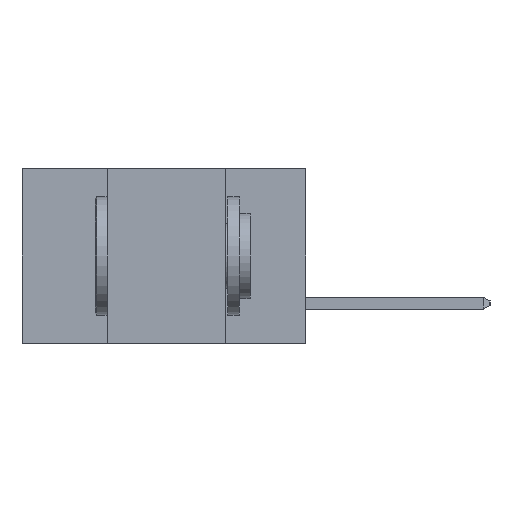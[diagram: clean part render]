
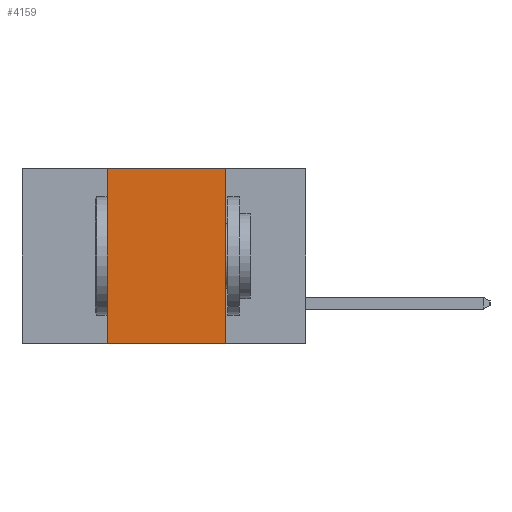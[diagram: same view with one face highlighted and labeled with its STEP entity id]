
A CAD part, left-side view. The second image highlights one B-rep face of the part: STEP entity #4159.
In plain terms, the highlighted planar face has unit normal (-1, 0, 0).
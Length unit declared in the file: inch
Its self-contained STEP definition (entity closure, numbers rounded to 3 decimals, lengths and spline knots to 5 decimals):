
#838 = LINE ( 'NONE', #1843, #7026 ) ;
#946 = VERTEX_POINT ( 'NONE', #10198 ) ;
#1693 = EDGE_LOOP ( 'NONE', ( #8256, #3713, #6201, #6331 ) ) ;
#1843 = CARTESIAN_POINT ( 'NONE',  ( 0., 0.42, -0.37 ) ) ;
#2211 = VECTOR ( 'NONE', #10298, 39.37008 ) ;
#2340 = FACE_OUTER_BOUND ( 'NONE', #1693, .T. ) ;
#2590 = EDGE_CURVE ( 'NONE', #2599, #5293, #3431, .T. ) ;
#2599 = VERTEX_POINT ( 'NONE', #6223 ) ;
#2770 = CARTESIAN_POINT ( 'NONE',  ( 0., 0.6, -0.37 ) ) ;
#3431 = LINE ( 'NONE', #5619, #5638 ) ;
#3527 = LINE ( 'NONE', #8804, #9727 ) ;
#3713 = ORIENTED_EDGE ( 'NONE', *, *, #2590, .F. ) ;
#3935 = EDGE_CURVE ( 'NONE', #946, #4389, #6920, .T. ) ;
#3956 = DIRECTION ( 'NONE',  ( 0., 0., -1. ) ) ;
#4159 = ADVANCED_FACE ( 'NONE', ( #2340 ), #9357, .F. ) ;
#4389 = VERTEX_POINT ( 'NONE', #6644 ) ;
#4640 = CARTESIAN_POINT ( 'NONE',  ( 0., 0.17, 0. ) ) ;
#5056 = EDGE_CURVE ( 'NONE', #946, #2599, #838, .T. ) ;
#5293 = VERTEX_POINT ( 'NONE', #4640 ) ;
#5400 = EDGE_CURVE ( 'NONE', #5293, #4389, #3527, .T. ) ;
#5619 = CARTESIAN_POINT ( 'NONE',  ( 0., 0.6, 0. ) ) ;
#5638 = VECTOR ( 'NONE', #7834, 39.37008 ) ;
#6201 = ORIENTED_EDGE ( 'NONE', *, *, #5056, .F. ) ;
#6223 = CARTESIAN_POINT ( 'NONE',  ( 0., 0.42, 0. ) ) ;
#6331 = ORIENTED_EDGE ( 'NONE', *, *, #3935, .T. ) ;
#6644 = CARTESIAN_POINT ( 'NONE',  ( 0., 0.17, -0.37 ) ) ;
#6915 = AXIS2_PLACEMENT_3D ( 'NONE', #9585, #9263, #9413 ) ;
#6920 = LINE ( 'NONE', #2770, #2211 ) ;
#7026 = VECTOR ( 'NONE', #9230, 39.37008 ) ;
#7834 = DIRECTION ( 'NONE',  ( 0., -1., 0. ) ) ;
#8256 = ORIENTED_EDGE ( 'NONE', *, *, #5400, .F. ) ;
#8804 = CARTESIAN_POINT ( 'NONE',  ( 0., 0.17, -0.37 ) ) ;
#9230 = DIRECTION ( 'NONE',  ( 0., 0., 1. ) ) ;
#9263 = DIRECTION ( 'NONE',  ( 1., 0., 0. ) ) ;
#9357 = PLANE ( 'NONE',  #6915 ) ;
#9413 = DIRECTION ( 'NONE',  ( 0., 0., -1. ) ) ;
#9585 = CARTESIAN_POINT ( 'NONE',  ( 0., 0.6, 0. ) ) ;
#9727 = VECTOR ( 'NONE', #3956, 39.37008 ) ;
#10198 = CARTESIAN_POINT ( 'NONE',  ( 0., 0.42, -0.37 ) ) ;
#10298 = DIRECTION ( 'NONE',  ( 0., -1., 0. ) ) ;
